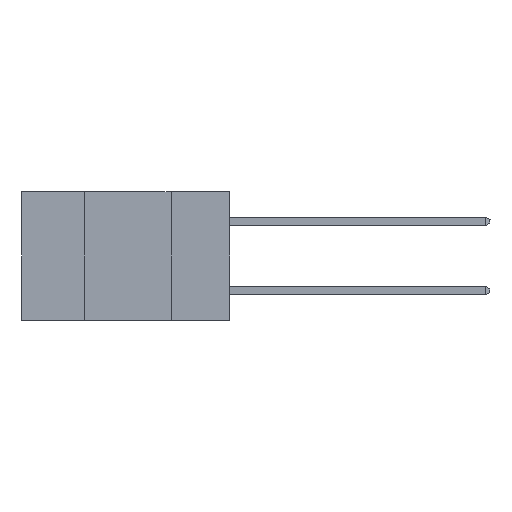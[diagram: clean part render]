
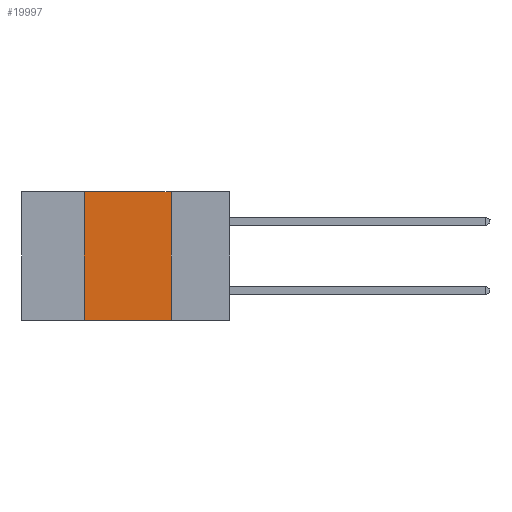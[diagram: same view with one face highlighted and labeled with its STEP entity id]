
A CAD part, left-side view. The second image highlights one B-rep face of the part: STEP entity #19997.
In plain terms, the highlighted planar face has unit normal (-1, 0, 0).
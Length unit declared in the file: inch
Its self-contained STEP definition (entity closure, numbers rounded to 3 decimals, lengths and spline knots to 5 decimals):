
#489 = VECTOR ( 'NONE', #24869, 39.37008 ) ;
#1989 = VERTEX_POINT ( 'NONE', #20499 ) ;
#2892 = FACE_OUTER_BOUND ( 'NONE', #14522, .T. ) ;
#3083 = LINE ( 'NONE', #13737, #22475 ) ;
#4065 = CARTESIAN_POINT ( 'NONE',  ( 0., 0.17, -0.37 ) ) ;
#4076 = LINE ( 'NONE', #7544, #15927 ) ;
#5906 = ORIENTED_EDGE ( 'NONE', *, *, #30737, .T. ) ;
#6428 = DIRECTION ( 'NONE',  ( 0., 0., -1. ) ) ;
#7248 = LINE ( 'NONE', #17141, #489 ) ;
#7544 = CARTESIAN_POINT ( 'NONE',  ( 0., 0.6, 0. ) ) ;
#9437 = PLANE ( 'NONE',  #18686 ) ;
#10768 = VECTOR ( 'NONE', #6428, 39.37008 ) ;
#11890 = ORIENTED_EDGE ( 'NONE', *, *, #20608, .F. ) ;
#11968 = DIRECTION ( 'NONE',  ( 1., 0., 0. ) ) ;
#13737 = CARTESIAN_POINT ( 'NONE',  ( 0., 0.42, 0. ) ) ;
#14522 = EDGE_LOOP ( 'NONE', ( #11890, #14699, #19788, #5906 ) ) ;
#14699 = ORIENTED_EDGE ( 'NONE', *, *, #20176, .F. ) ;
#15050 = DIRECTION ( 'NONE',  ( 0., -1., 0. ) ) ;
#15352 = VERTEX_POINT ( 'NONE', #4065 ) ;
#15927 = VECTOR ( 'NONE', #15050, 39.37008 ) ;
#16294 = DIRECTION ( 'NONE',  ( 0., 0., 1. ) ) ;
#16586 = CARTESIAN_POINT ( 'NONE',  ( 0., 0.17, 0. ) ) ;
#16700 = LINE ( 'NONE', #16586, #10768 ) ;
#17141 = CARTESIAN_POINT ( 'NONE',  ( 0., 0.6, -0.37 ) ) ;
#18686 = AXIS2_PLACEMENT_3D ( 'NONE', #27119, #11968, #29644 ) ;
#19250 = CARTESIAN_POINT ( 'NONE',  ( 0., 0.42, -0.37 ) ) ;
#19788 = ORIENTED_EDGE ( 'NONE', *, *, #27366, .F. ) ;
#19997 = ADVANCED_FACE ( 'NONE', ( #2892 ), #9437, .F. ) ;
#20176 = EDGE_CURVE ( 'NONE', #1989, #24634, #4076, .T. ) ;
#20499 = CARTESIAN_POINT ( 'NONE',  ( 0., 0.42, 0. ) ) ;
#20608 = EDGE_CURVE ( 'NONE', #24634, #15352, #16700, .T. ) ;
#20661 = VERTEX_POINT ( 'NONE', #19250 ) ;
#22218 = CARTESIAN_POINT ( 'NONE',  ( 0., 0.17, 0. ) ) ;
#22475 = VECTOR ( 'NONE', #16294, 39.37008 ) ;
#24634 = VERTEX_POINT ( 'NONE', #22218 ) ;
#24869 = DIRECTION ( 'NONE',  ( 0., -1., 0. ) ) ;
#27119 = CARTESIAN_POINT ( 'NONE',  ( 0., 0.6, 0. ) ) ;
#27366 = EDGE_CURVE ( 'NONE', #20661, #1989, #3083, .T. ) ;
#29644 = DIRECTION ( 'NONE',  ( 0., 0., -1. ) ) ;
#30737 = EDGE_CURVE ( 'NONE', #20661, #15352, #7248, .T. ) ;
